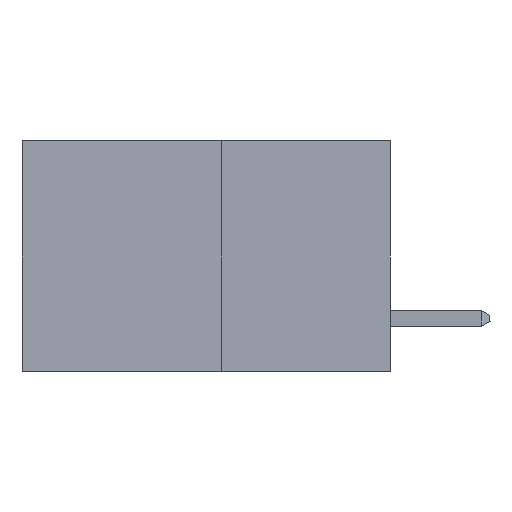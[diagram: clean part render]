
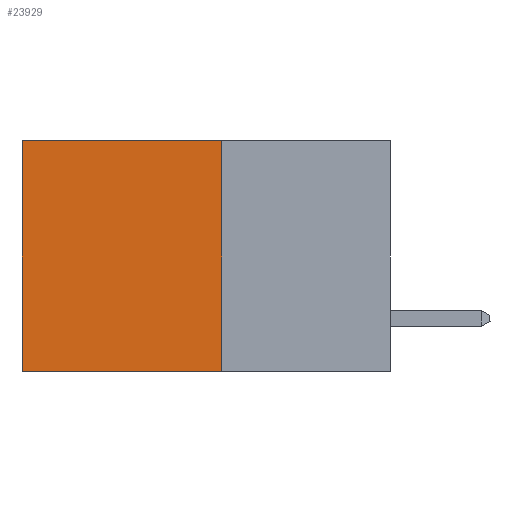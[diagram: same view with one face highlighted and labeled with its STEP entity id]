
A CAD part, left-side view. The second image highlights one B-rep face of the part: STEP entity #23929.
In plain terms, the highlighted planar face has unit normal (-1, 0, 0).
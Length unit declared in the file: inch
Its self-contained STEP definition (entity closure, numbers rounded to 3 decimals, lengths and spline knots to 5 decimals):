
#667 = CARTESIAN_POINT ( 'NONE',  ( 0.277, 0.27, -0.37 ) ) ;
#1355 = CARTESIAN_POINT ( 'NONE',  ( 0.277, 0.27, -0.37 ) ) ;
#3339 = ORIENTED_EDGE ( 'NONE', *, *, #15653, .F. ) ;
#3449 = VERTEX_POINT ( 'NONE', #13538 ) ;
#3586 = EDGE_CURVE ( 'NONE', #20425, #5074, #18033, .T. ) ;
#3792 = LINE ( 'NONE', #1355, #14519 ) ;
#4252 = DIRECTION ( 'NONE',  ( 0., 1., 0. ) ) ;
#4780 = FACE_OUTER_BOUND ( 'NONE', #27684, .T. ) ;
#5074 = VERTEX_POINT ( 'NONE', #10458 ) ;
#5962 = CARTESIAN_POINT ( 'NONE',  ( 0.277, 0.27, 0. ) ) ;
#9108 = VECTOR ( 'NONE', #11807, 39.37008 ) ;
#9337 = CARTESIAN_POINT ( 'NONE',  ( 0.277, 0.59, -0.37 ) ) ;
#10458 = CARTESIAN_POINT ( 'NONE',  ( 0.277, 0.59, 0. ) ) ;
#10814 = VECTOR ( 'NONE', #27551, 39.37008 ) ;
#11365 = DIRECTION ( 'NONE',  ( 0., 0., -1. ) ) ;
#11807 = DIRECTION ( 'NONE',  ( 0., 0., -1. ) ) ;
#13115 = CARTESIAN_POINT ( 'NONE',  ( 0.277, 0.27, 0. ) ) ;
#13449 = DIRECTION ( 'NONE',  ( 1., 0., 0. ) ) ;
#13538 = CARTESIAN_POINT ( 'NONE',  ( 0.277, 0.27, -0.37 ) ) ;
#14519 = VECTOR ( 'NONE', #11365, 39.37008 ) ;
#15653 = EDGE_CURVE ( 'NONE', #20425, #3449, #3792, .T. ) ;
#18033 = LINE ( 'NONE', #5962, #23653 ) ;
#18157 = LINE ( 'NONE', #667, #10814 ) ;
#18931 = AXIS2_PLACEMENT_3D ( 'NONE', #27907, #13449, #30284 ) ;
#19156 = EDGE_CURVE ( 'NONE', #3449, #26020, #18157, .T. ) ;
#20425 = VERTEX_POINT ( 'NONE', #13115 ) ;
#20716 = PLANE ( 'NONE',  #18931 ) ;
#21310 = ORIENTED_EDGE ( 'NONE', *, *, #31402, .T. ) ;
#22438 = ORIENTED_EDGE ( 'NONE', *, *, #3586, .T. ) ;
#23653 = VECTOR ( 'NONE', #4252, 39.37008 ) ;
#23929 = ADVANCED_FACE ( 'NONE', ( #4780 ), #20716, .F. ) ;
#26020 = VERTEX_POINT ( 'NONE', #26531 ) ;
#26531 = CARTESIAN_POINT ( 'NONE',  ( 0.277, 0.59, -0.37 ) ) ;
#27551 = DIRECTION ( 'NONE',  ( 0., 1., 0. ) ) ;
#27684 = EDGE_LOOP ( 'NONE', ( #21310, #30301, #3339, #22438 ) ) ;
#27907 = CARTESIAN_POINT ( 'NONE',  ( 0.277, 0.27, -0.37 ) ) ;
#28414 = LINE ( 'NONE', #9337, #9108 ) ;
#30284 = DIRECTION ( 'NONE',  ( 0., 0., -1. ) ) ;
#30301 = ORIENTED_EDGE ( 'NONE', *, *, #19156, .F. ) ;
#31402 = EDGE_CURVE ( 'NONE', #5074, #26020, #28414, .T. ) ;
